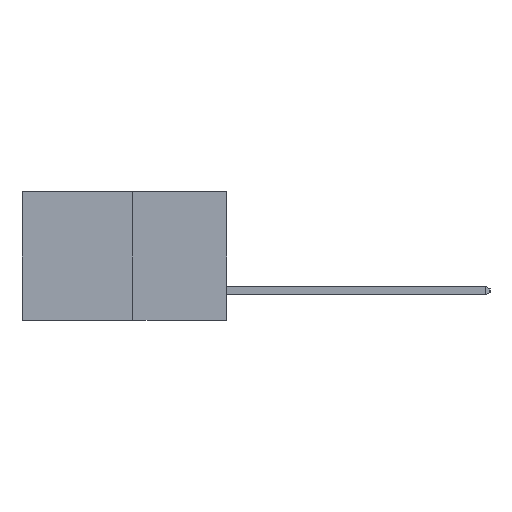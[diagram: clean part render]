
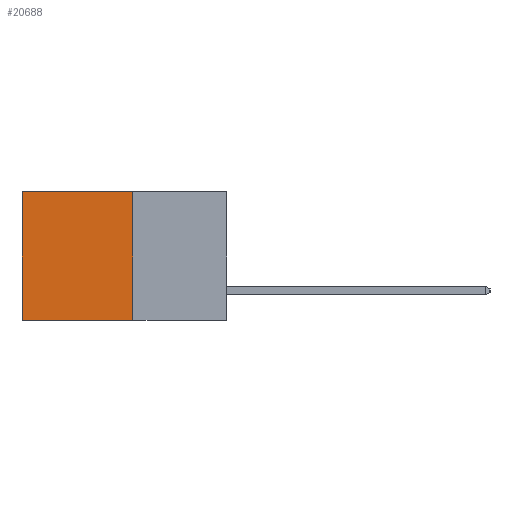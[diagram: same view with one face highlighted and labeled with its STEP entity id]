
A CAD part, left-side view. The second image highlights one B-rep face of the part: STEP entity #20688.
In plain terms, the highlighted planar face has unit normal (-1, 0, 0).
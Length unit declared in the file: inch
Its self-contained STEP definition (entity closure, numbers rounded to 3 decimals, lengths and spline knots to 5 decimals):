
#542 = VERTEX_POINT ( 'NONE', #10838 ) ;
#3279 = EDGE_LOOP ( 'NONE', ( #7449, #11998, #19907, #24562 ) ) ;
#3536 = EDGE_CURVE ( 'NONE', #15111, #8309, #14071, .T. ) ;
#3645 = VECTOR ( 'NONE', #10156, 39.37008 ) ;
#3976 = CARTESIAN_POINT ( 'NONE',  ( 0.277, 0.59, 0. ) ) ;
#4286 = VECTOR ( 'NONE', #5693, 39.37008 ) ;
#5693 = DIRECTION ( 'NONE',  ( 0., 1., 0. ) ) ;
#7449 = ORIENTED_EDGE ( 'NONE', *, *, #21468, .T. ) ;
#7795 = CARTESIAN_POINT ( 'NONE',  ( 0.277, 0.27, -0.37 ) ) ;
#8309 = VERTEX_POINT ( 'NONE', #22542 ) ;
#8464 = DIRECTION ( 'NONE',  ( 1., 0., 0. ) ) ;
#9581 = VECTOR ( 'NONE', #11702, 39.37008 ) ;
#9953 = CARTESIAN_POINT ( 'NONE',  ( 0.277, 0.27, 0. ) ) ;
#10151 = LINE ( 'NONE', #19198, #4286 ) ;
#10156 = DIRECTION ( 'NONE',  ( 0., 0., -1. ) ) ;
#10838 = CARTESIAN_POINT ( 'NONE',  ( 0.277, 0.59, -0.37 ) ) ;
#11702 = DIRECTION ( 'NONE',  ( 0., 1., 0. ) ) ;
#11998 = ORIENTED_EDGE ( 'NONE', *, *, #23963, .F. ) ;
#12286 = PLANE ( 'NONE',  #20816 ) ;
#13008 = DIRECTION ( 'NONE',  ( 0., 0., -1. ) ) ;
#13687 = FACE_OUTER_BOUND ( 'NONE', #3279, .T. ) ;
#14071 = LINE ( 'NONE', #15225, #3645 ) ;
#14713 = LINE ( 'NONE', #7795, #9581 ) ;
#15111 = VERTEX_POINT ( 'NONE', #9953 ) ;
#15225 = CARTESIAN_POINT ( 'NONE',  ( 0.277, 0.27, -0.37 ) ) ;
#17013 = VERTEX_POINT ( 'NONE', #3976 ) ;
#18148 = EDGE_CURVE ( 'NONE', #15111, #17013, #10151, .T. ) ;
#18713 = LINE ( 'NONE', #22533, #23218 ) ;
#19198 = CARTESIAN_POINT ( 'NONE',  ( 0.277, 0.27, 0. ) ) ;
#19907 = ORIENTED_EDGE ( 'NONE', *, *, #3536, .F. ) ;
#19977 = CARTESIAN_POINT ( 'NONE',  ( 0.277, 0.27, -0.37 ) ) ;
#20688 = ADVANCED_FACE ( 'NONE', ( #13687 ), #12286, .F. ) ;
#20816 = AXIS2_PLACEMENT_3D ( 'NONE', #19977, #8464, #21902 ) ;
#21468 = EDGE_CURVE ( 'NONE', #17013, #542, #18713, .T. ) ;
#21902 = DIRECTION ( 'NONE',  ( 0., 0., -1. ) ) ;
#22533 = CARTESIAN_POINT ( 'NONE',  ( 0.277, 0.59, -0.37 ) ) ;
#22542 = CARTESIAN_POINT ( 'NONE',  ( 0.277, 0.27, -0.37 ) ) ;
#23218 = VECTOR ( 'NONE', #13008, 39.37008 ) ;
#23963 = EDGE_CURVE ( 'NONE', #8309, #542, #14713, .T. ) ;
#24562 = ORIENTED_EDGE ( 'NONE', *, *, #18148, .T. ) ;
